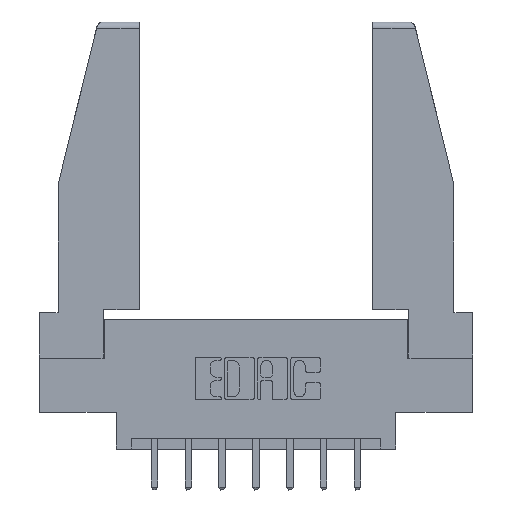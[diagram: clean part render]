
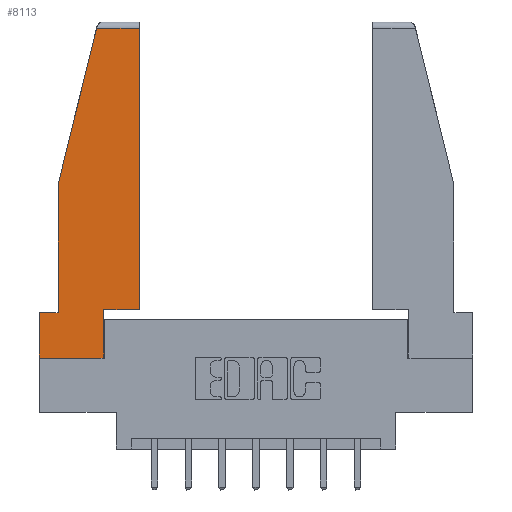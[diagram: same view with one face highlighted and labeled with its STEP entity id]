
A CAD part, top view. The second image highlights one B-rep face of the part: STEP entity #8113.
In plain terms, the highlighted planar face has unit normal (0, 0, 1).
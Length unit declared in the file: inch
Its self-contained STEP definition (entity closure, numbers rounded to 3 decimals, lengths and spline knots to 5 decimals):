
#768 = LINE ( 'NONE', #11266, #9498 ) ;
#833 = ORIENTED_EDGE ( 'NONE', *, *, #11888, .T. ) ;
#897 = EDGE_CURVE ( 'NONE', #7776, #12155, #3589, .T. ) ;
#1763 = DIRECTION ( 'NONE',  ( 1., 0., 0. ) ) ;
#2116 = EDGE_LOOP ( 'NONE', ( #10068, #833, #7593, #3093, #2347, #4954, #9176, #5688, #3518 ) ) ;
#2277 = EDGE_CURVE ( 'NONE', #6614, #8927, #6750, .T. ) ;
#2347 = ORIENTED_EDGE ( 'NONE', *, *, #897, .T. ) ;
#2441 = EDGE_CURVE ( 'NONE', #6484, #6614, #11008, .T. ) ;
#2503 = CARTESIAN_POINT ( 'NONE',  ( 0.086, 0.8, 0. ) ) ;
#2714 = VECTOR ( 'NONE', #12217, 39.37008 ) ;
#2773 = AXIS2_PLACEMENT_3D ( 'NONE', #4592, #10479, #1763 ) ;
#3093 = ORIENTED_EDGE ( 'NONE', *, *, #7546, .T. ) ;
#3227 = DIRECTION ( 'NONE',  ( -1., 0., 0. ) ) ;
#3493 = LINE ( 'NONE', #4903, #10791 ) ;
#3518 = ORIENTED_EDGE ( 'NONE', *, *, #2441, .T. ) ;
#3575 = DIRECTION ( 'NONE',  ( -0.239, -0.971, 0. ) ) ;
#3589 = LINE ( 'NONE', #4995, #8795 ) ;
#3613 = CARTESIAN_POINT ( 'NONE',  ( 0., 0.21, 0. ) ) ;
#3632 = CARTESIAN_POINT ( 'NONE',  ( 0.297, 0.223, 0. ) ) ;
#3914 = CARTESIAN_POINT ( 'NONE',  ( 0., 0., 0. ) ) ;
#4481 = EDGE_CURVE ( 'NONE', #8245, #5151, #6262, .T. ) ;
#4575 = CARTESIAN_POINT ( 'NONE',  ( 0.297, 0., 0. ) ) ;
#4586 = DIRECTION ( 'NONE',  ( 1., 0., 0. ) ) ;
#4592 = CARTESIAN_POINT ( 'NONE',  ( 0., 0., 0. ) ) ;
#4817 = LINE ( 'NONE', #4575, #2714 ) ;
#4894 = VECTOR ( 'NONE', #9547, 39.37008 ) ;
#4903 = CARTESIAN_POINT ( 'NONE',  ( 0.086, 0.8, 0. ) ) ;
#4954 = ORIENTED_EDGE ( 'NONE', *, *, #4959, .T. ) ;
#4959 = EDGE_CURVE ( 'NONE', #12155, #8245, #10819, .T. ) ;
#4995 = CARTESIAN_POINT ( 'NONE',  ( 0., 0.21, 0. ) ) ;
#5151 = VERTEX_POINT ( 'NONE', #6865 ) ;
#5491 = DIRECTION ( 'NONE',  ( 0., 1., 0. ) ) ;
#5688 = ORIENTED_EDGE ( 'NONE', *, *, #8666, .T. ) ;
#5822 = DIRECTION ( 'NONE',  ( 0., -1., 0. ) ) ;
#5857 = DIRECTION ( 'NONE',  ( 0., -1., 0. ) ) ;
#6190 = VECTOR ( 'NONE', #3227, 39.37008 ) ;
#6262 = LINE ( 'NONE', #11502, #4894 ) ;
#6326 = EDGE_CURVE ( 'NONE', #6926, #10593, #768, .T. ) ;
#6484 = VERTEX_POINT ( 'NONE', #10661 ) ;
#6614 = VERTEX_POINT ( 'NONE', #11772 ) ;
#6711 = CARTESIAN_POINT ( 'NONE',  ( 0., 0.21, 0. ) ) ;
#6750 = LINE ( 'NONE', #12424, #10254 ) ;
#6865 = CARTESIAN_POINT ( 'NONE',  ( 0.297, 0., 0. ) ) ;
#6926 = VERTEX_POINT ( 'NONE', #7754 ) ;
#7325 = VECTOR ( 'NONE', #5822, 39.37008 ) ;
#7546 = EDGE_CURVE ( 'NONE', #10593, #7776, #3493, .T. ) ;
#7557 = DIRECTION ( 'NONE',  ( -1., 0., 0. ) ) ;
#7593 = ORIENTED_EDGE ( 'NONE', *, *, #6326, .T. ) ;
#7754 = CARTESIAN_POINT ( 'NONE',  ( 0.2636, 1.52, 0. ) ) ;
#7776 = VERTEX_POINT ( 'NONE', #11079 ) ;
#8104 = CARTESIAN_POINT ( 'NONE',  ( 0., 1.52, 0. ) ) ;
#8113 = ADVANCED_FACE ( 'NONE', ( #11876 ), #10527, .T. ) ;
#8245 = VERTEX_POINT ( 'NONE', #3914 ) ;
#8666 = EDGE_CURVE ( 'NONE', #5151, #6484, #4817, .T. ) ;
#8795 = VECTOR ( 'NONE', #7557, 39.37008 ) ;
#8926 = CARTESIAN_POINT ( 'NONE',  ( 0.461, 1.52, 0. ) ) ;
#8927 = VERTEX_POINT ( 'NONE', #8926 ) ;
#9176 = ORIENTED_EDGE ( 'NONE', *, *, #4481, .T. ) ;
#9498 = VECTOR ( 'NONE', #3575, 39.37008 ) ;
#9547 = DIRECTION ( 'NONE',  ( 1., 0., 0. ) ) ;
#10068 = ORIENTED_EDGE ( 'NONE', *, *, #2277, .T. ) ;
#10163 = LINE ( 'NONE', #8104, #6190 ) ;
#10254 = VECTOR ( 'NONE', #5491, 39.37008 ) ;
#10479 = DIRECTION ( 'NONE',  ( 0., 0., 1. ) ) ;
#10527 = PLANE ( 'NONE',  #2773 ) ;
#10593 = VERTEX_POINT ( 'NONE', #2503 ) ;
#10661 = CARTESIAN_POINT ( 'NONE',  ( 0.297, 0.223, 0. ) ) ;
#10791 = VECTOR ( 'NONE', #5857, 39.37008 ) ;
#10819 = LINE ( 'NONE', #6711, #7325 ) ;
#11008 = LINE ( 'NONE', #3632, #11168 ) ;
#11079 = CARTESIAN_POINT ( 'NONE',  ( 0.086, 0.21, 0. ) ) ;
#11168 = VECTOR ( 'NONE', #4586, 39.37008 ) ;
#11266 = CARTESIAN_POINT ( 'NONE',  ( 0.271, 1.55, 0. ) ) ;
#11502 = CARTESIAN_POINT ( 'NONE',  ( 0., 0., 0. ) ) ;
#11772 = CARTESIAN_POINT ( 'NONE',  ( 0.461, 0.223, 0. ) ) ;
#11876 = FACE_OUTER_BOUND ( 'NONE', #2116, .T. ) ;
#11888 = EDGE_CURVE ( 'NONE', #8927, #6926, #10163, .T. ) ;
#12155 = VERTEX_POINT ( 'NONE', #3613 ) ;
#12217 = DIRECTION ( 'NONE',  ( 0., 1., 0. ) ) ;
#12424 = CARTESIAN_POINT ( 'NONE',  ( 0.461, 0.223, 0. ) ) ;
